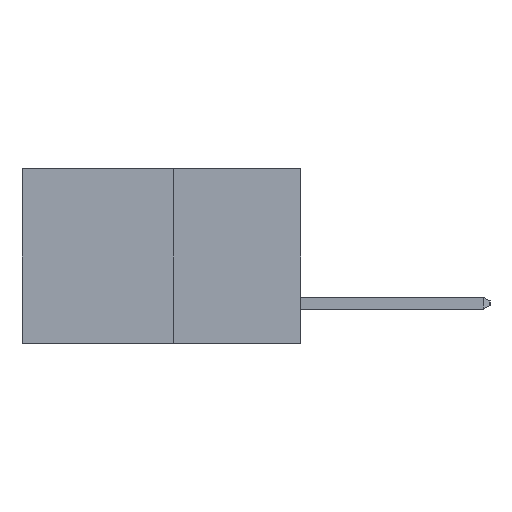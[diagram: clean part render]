
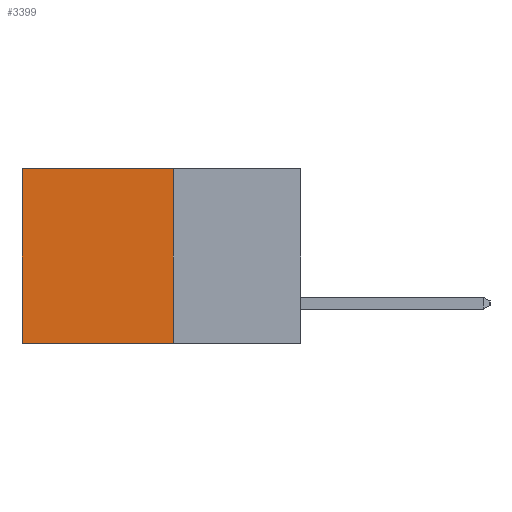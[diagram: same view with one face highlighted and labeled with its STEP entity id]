
A CAD part, left-side view. The second image highlights one B-rep face of the part: STEP entity #3399.
In plain terms, the highlighted planar face has unit normal (-1, 0, 0).
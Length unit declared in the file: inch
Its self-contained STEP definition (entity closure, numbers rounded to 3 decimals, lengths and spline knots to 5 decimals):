
#28 = ORIENTED_EDGE ( 'NONE', *, *, #8319, .F. ) ;
#523 = VECTOR ( 'NONE', #8009, 39.37008 ) ;
#640 = ORIENTED_EDGE ( 'NONE', *, *, #1083, .T. ) ;
#802 = EDGE_CURVE ( 'NONE', #5294, #4461, #8706, .T. ) ;
#1083 = EDGE_CURVE ( 'NONE', #4799, #5294, #8822, .T. ) ;
#1194 = CARTESIAN_POINT ( 'NONE',  ( 0.277, 0.59, -0.37 ) ) ;
#1221 = CARTESIAN_POINT ( 'NONE',  ( 0.277, 0.27, 0. ) ) ;
#1415 = LINE ( 'NONE', #5787, #9343 ) ;
#2123 = LINE ( 'NONE', #5234, #6114 ) ;
#3323 = DIRECTION ( 'NONE',  ( 0., 0., -1. ) ) ;
#3399 = ADVANCED_FACE ( 'NONE', ( #9268 ), #4428, .F. ) ;
#3804 = CARTESIAN_POINT ( 'NONE',  ( 0.277, 0.27, -0.37 ) ) ;
#4257 = DIRECTION ( 'NONE',  ( 0., 0., -1. ) ) ;
#4384 = DIRECTION ( 'NONE',  ( 1., 0., 0. ) ) ;
#4425 = AXIS2_PLACEMENT_3D ( 'NONE', #4643, #4384, #4257 ) ;
#4428 = PLANE ( 'NONE',  #4425 ) ;
#4461 = VERTEX_POINT ( 'NONE', #7767 ) ;
#4513 = EDGE_LOOP ( 'NONE', ( #8338, #28, #6446, #640 ) ) ;
#4643 = CARTESIAN_POINT ( 'NONE',  ( 0.277, 0.27, -0.37 ) ) ;
#4799 = VERTEX_POINT ( 'NONE', #1221 ) ;
#5008 = DIRECTION ( 'NONE',  ( 0., 0., -1. ) ) ;
#5234 = CARTESIAN_POINT ( 'NONE',  ( 0.277, 0.27, -0.37 ) ) ;
#5294 = VERTEX_POINT ( 'NONE', #6958 ) ;
#5787 = CARTESIAN_POINT ( 'NONE',  ( 0.277, 0.27, -0.37 ) ) ;
#6114 = VECTOR ( 'NONE', #8253, 39.37008 ) ;
#6446 = ORIENTED_EDGE ( 'NONE', *, *, #8171, .F. ) ;
#6643 = VECTOR ( 'NONE', #3323, 39.37008 ) ;
#6958 = CARTESIAN_POINT ( 'NONE',  ( 0.277, 0.59, 0. ) ) ;
#7767 = CARTESIAN_POINT ( 'NONE',  ( 0.277, 0.59, -0.37 ) ) ;
#8009 = DIRECTION ( 'NONE',  ( 0., 1., 0. ) ) ;
#8171 = EDGE_CURVE ( 'NONE', #4799, #8514, #1415, .T. ) ;
#8253 = DIRECTION ( 'NONE',  ( 0., 1., 0. ) ) ;
#8319 = EDGE_CURVE ( 'NONE', #8514, #4461, #2123, .T. ) ;
#8338 = ORIENTED_EDGE ( 'NONE', *, *, #802, .T. ) ;
#8514 = VERTEX_POINT ( 'NONE', #3804 ) ;
#8629 = CARTESIAN_POINT ( 'NONE',  ( 0.277, 0.27, 0. ) ) ;
#8706 = LINE ( 'NONE', #1194, #6643 ) ;
#8822 = LINE ( 'NONE', #8629, #523 ) ;
#9268 = FACE_OUTER_BOUND ( 'NONE', #4513, .T. ) ;
#9343 = VECTOR ( 'NONE', #5008, 39.37008 ) ;
